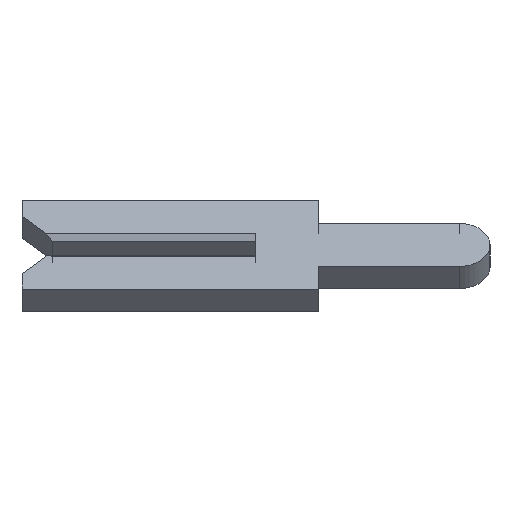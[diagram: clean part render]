
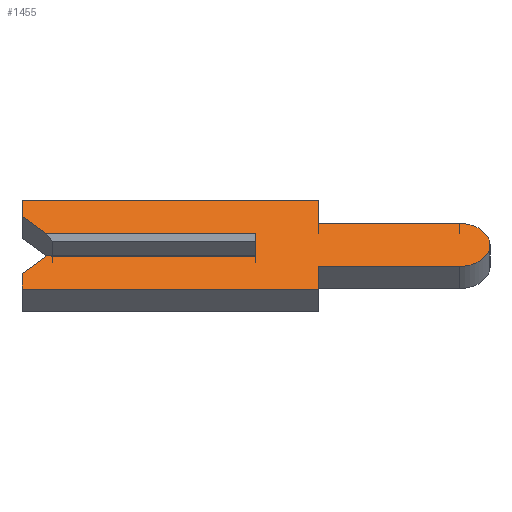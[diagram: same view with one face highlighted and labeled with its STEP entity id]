
A CAD part, left-side view. The second image highlights one B-rep face of the part: STEP entity #1455.
In plain terms, the highlighted face is planar.
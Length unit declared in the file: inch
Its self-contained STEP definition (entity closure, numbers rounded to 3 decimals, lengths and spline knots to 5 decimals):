
#9 = CARTESIAN_POINT ( 'NONE',  ( -0.01, 0.1305, 0.0065 ) ) ;
#16 = VERTEX_POINT ( 'NONE', #1752 ) ;
#35 = VECTOR ( 'NONE', #376, 39.37008 ) ;
#37 = CARTESIAN_POINT ( 'NONE',  ( -0.01, 0.134, 0.01 ) ) ;
#63 = DIRECTION ( 'NONE',  ( 0., -1., 0. ) ) ;
#74 = ORIENTED_EDGE ( 'NONE', *, *, #1383, .F. ) ;
#86 = CARTESIAN_POINT ( 'NONE',  ( -0.01, -0.04, -0.04 ) ) ;
#107 = EDGE_CURVE ( 'NONE', #1207, #773, #765, .T. ) ;
#119 = DIRECTION ( 'NONE',  ( 0., 0., 1. ) ) ;
#122 = AXIS2_PLACEMENT_3D ( 'NONE', #515, #1673, #805 ) ;
#140 = DIRECTION ( 'NONE',  ( 0., 0.707, 0.707 ) ) ;
#144 = CARTESIAN_POINT ( 'NONE',  ( -0.01, -0.04, 0.0195 ) ) ;
#207 = CARTESIAN_POINT ( 'NONE',  ( -0.01, 0.15, 0.026 ) ) ;
#211 = EDGE_CURVE ( 'NONE', #896, #400, #517, .T. ) ;
#214 = CARTESIAN_POINT ( 'NONE',  ( -0.01, 0.15, 0.01 ) ) ;
#222 = CARTESIAN_POINT ( 'NONE',  ( -0.01, -0.04, 0.0195 ) ) ;
#225 = LINE ( 'NONE', #992, #1012 ) ;
#232 = DIRECTION ( 'NONE',  ( 0., 0., -1. ) ) ;
#243 = VECTOR ( 'NONE', #232, 39.37008 ) ;
#244 = DIRECTION ( 'NONE',  ( 0., -0.707, 0.707 ) ) ;
#254 = ORIENTED_EDGE ( 'NONE', *, *, #1159, .F. ) ;
#257 = CARTESIAN_POINT ( 'NONE',  ( -0.01, 0.15, 0.04 ) ) ;
#262 = DIRECTION ( 'NONE',  ( 1., 0., 0. ) ) ;
#268 = VECTOR ( 'NONE', #952, 39.37008 ) ;
#288 = LINE ( 'NONE', #681, #630 ) ;
#320 = CARTESIAN_POINT ( 'NONE',  ( -0.01, 0.15, -0.026 ) ) ;
#349 = VERTEX_POINT ( 'NONE', #1772 ) ;
#360 = LINE ( 'NONE', #541, #1742 ) ;
#376 = DIRECTION ( 'NONE',  ( 0., 0., -1. ) ) ;
#378 = LINE ( 'NONE', #811, #268 ) ;
#397 = VECTOR ( 'NONE', #1154, 39.37008 ) ;
#400 = VERTEX_POINT ( 'NONE', #1021 ) ;
#404 = CARTESIAN_POINT ( 'NONE',  ( -0.01, -0.1305, 0. ) ) ;
#422 = LINE ( 'NONE', #795, #1818 ) ;
#462 = VERTEX_POINT ( 'NONE', #320 ) ;
#465 = VERTEX_POINT ( 'NONE', #1200 ) ;
#481 = CARTESIAN_POINT ( 'NONE',  ( -0.01, -0.04, -0.0195 ) ) ;
#515 = CARTESIAN_POINT ( 'NONE',  ( -0.01, -0.1305, 0. ) ) ;
#517 = LINE ( 'NONE', #9, #1617 ) ;
#521 = ORIENTED_EDGE ( 'NONE', *, *, #107, .F. ) ;
#541 = CARTESIAN_POINT ( 'NONE',  ( -0.01, 0.15, -0.026 ) ) ;
#549 = ORIENTED_EDGE ( 'NONE', *, *, #987, .T. ) ;
#559 = CARTESIAN_POINT ( 'NONE',  ( -0.01, -0.04, 0.04 ) ) ;
#609 = LINE ( 'NONE', #86, #243 ) ;
#623 = ORIENTED_EDGE ( 'NONE', *, *, #1677, .F. ) ;
#630 = VECTOR ( 'NONE', #997, 39.37008 ) ;
#668 = DIRECTION ( 'NONE',  ( 0., -1., 0. ) ) ;
#674 = LINE ( 'NONE', #222, #993 ) ;
#681 = CARTESIAN_POINT ( 'NONE',  ( -0.01, -0.04, -0.0195 ) ) ;
#692 = EDGE_LOOP ( 'NONE', ( #549, #1679, #749, #254, #623, #521, #959, #1429, #1628, #1826, #837, #74, #1052, #978 ) ) ;
#718 = VECTOR ( 'NONE', #244, 39.37008 ) ;
#720 = VECTOR ( 'NONE', #1498, 39.37008 ) ;
#749 = ORIENTED_EDGE ( 'NONE', *, *, #1249, .F. ) ;
#765 = LINE ( 'NONE', #1160, #397 ) ;
#773 = VERTEX_POINT ( 'NONE', #1509 ) ;
#792 = EDGE_CURVE ( 'NONE', #400, #1481, #830, .T. ) ;
#795 = CARTESIAN_POINT ( 'NONE',  ( -0.01, -0.1305, -0.01 ) ) ;
#805 = DIRECTION ( 'NONE',  ( 0., 0., -1. ) ) ;
#811 = CARTESIAN_POINT ( 'NONE',  ( -0.01, 0.15, 0.04 ) ) ;
#830 = LINE ( 'NONE', #207, #720 ) ;
#837 = ORIENTED_EDGE ( 'NONE', *, *, #1413, .F. ) ;
#863 = VERTEX_POINT ( 'NONE', #1655 ) ;
#896 = VERTEX_POINT ( 'NONE', #37 ) ;
#900 = LINE ( 'NONE', #1252, #35 ) ;
#912 = AXIS2_PLACEMENT_3D ( 'NONE', #404, #262, #1568 ) ;
#952 = DIRECTION ( 'NONE',  ( 0., -1., 0. ) ) ;
#956 = DIRECTION ( 'NONE',  ( 0., -1., 0. ) ) ;
#959 = ORIENTED_EDGE ( 'NONE', *, *, #1449, .F. ) ;
#978 = ORIENTED_EDGE ( 'NONE', *, *, #211, .F. ) ;
#987 = EDGE_CURVE ( 'NONE', #896, #1494, #1202, .T. ) ;
#992 = CARTESIAN_POINT ( 'NONE',  ( -0.01, 0., 0.0065 ) ) ;
#993 = VECTOR ( 'NONE', #668, 39.37008 ) ;
#997 = DIRECTION ( 'NONE',  ( 0., 1., 0. ) ) ;
#1012 = VECTOR ( 'NONE', #119, 39.37008 ) ;
#1021 = CARTESIAN_POINT ( 'NONE',  ( -0.01, 0.15, 0.026 ) ) ;
#1052 = ORIENTED_EDGE ( 'NONE', *, *, #792, .F. ) ;
#1079 = VECTOR ( 'NONE', #63, 39.37008 ) ;
#1097 = VERTEX_POINT ( 'NONE', #481 ) ;
#1153 = CIRCLE ( 'NONE', #122, 0.0195 ) ;
#1154 = DIRECTION ( 'NONE',  ( 0., 1., 0. ) ) ;
#1159 = EDGE_CURVE ( 'NONE', #462, #465, #1682, .T. ) ;
#1160 = CARTESIAN_POINT ( 'NONE',  ( -0.01, 0.15, -0.04 ) ) ;
#1170 = VERTEX_POINT ( 'NONE', #144 ) ;
#1200 = CARTESIAN_POINT ( 'NONE',  ( -0.01, 0.134, -0.01 ) ) ;
#1202 = LINE ( 'NONE', #214, #1079 ) ;
#1207 = VERTEX_POINT ( 'NONE', #1685 ) ;
#1222 = EDGE_CURVE ( 'NONE', #863, #349, #1153, .T. ) ;
#1249 = EDGE_CURVE ( 'NONE', #465, #16, #422, .T. ) ;
#1252 = CARTESIAN_POINT ( 'NONE',  ( -0.01, -0.04, 0.04 ) ) ;
#1383 = EDGE_CURVE ( 'NONE', #1481, #1686, #378, .T. ) ;
#1411 = PLANE ( 'NONE',  #912 ) ;
#1413 = EDGE_CURVE ( 'NONE', #1686, #1170, #900, .T. ) ;
#1429 = ORIENTED_EDGE ( 'NONE', *, *, #1583, .F. ) ;
#1434 = EDGE_CURVE ( 'NONE', #1170, #863, #674, .T. ) ;
#1449 = EDGE_CURVE ( 'NONE', #1097, #1207, #609, .T. ) ;
#1455 = ADVANCED_FACE ( 'NONE', ( #1797 ), #1411, .F. ) ;
#1481 = VERTEX_POINT ( 'NONE', #257 ) ;
#1494 = VERTEX_POINT ( 'NONE', #1726 ) ;
#1498 = DIRECTION ( 'NONE',  ( 0., 0., 1. ) ) ;
#1509 = CARTESIAN_POINT ( 'NONE',  ( -0.01, 0.15, -0.04 ) ) ;
#1519 = CARTESIAN_POINT ( 'NONE',  ( -0.01, 0.1305, -0.0065 ) ) ;
#1554 = EDGE_CURVE ( 'NONE', #16, #1494, #225, .T. ) ;
#1568 = DIRECTION ( 'NONE',  ( 0., 0., -1. ) ) ;
#1580 = DIRECTION ( 'NONE',  ( 0., 0., 1. ) ) ;
#1583 = EDGE_CURVE ( 'NONE', #349, #1097, #288, .T. ) ;
#1617 = VECTOR ( 'NONE', #140, 39.37008 ) ;
#1628 = ORIENTED_EDGE ( 'NONE', *, *, #1222, .F. ) ;
#1655 = CARTESIAN_POINT ( 'NONE',  ( -0.01, -0.1305, 0.0195 ) ) ;
#1673 = DIRECTION ( 'NONE',  ( 1., 0., 0. ) ) ;
#1677 = EDGE_CURVE ( 'NONE', #773, #462, #360, .T. ) ;
#1679 = ORIENTED_EDGE ( 'NONE', *, *, #1554, .F. ) ;
#1682 = LINE ( 'NONE', #1519, #718 ) ;
#1685 = CARTESIAN_POINT ( 'NONE',  ( -0.01, -0.04, -0.04 ) ) ;
#1686 = VERTEX_POINT ( 'NONE', #559 ) ;
#1726 = CARTESIAN_POINT ( 'NONE',  ( -0.01, 0., 0.01 ) ) ;
#1742 = VECTOR ( 'NONE', #1580, 39.37008 ) ;
#1752 = CARTESIAN_POINT ( 'NONE',  ( -0.01, 0., -0.01 ) ) ;
#1772 = CARTESIAN_POINT ( 'NONE',  ( -0.01, -0.1305, -0.0195 ) ) ;
#1797 = FACE_OUTER_BOUND ( 'NONE', #692, .T. ) ;
#1818 = VECTOR ( 'NONE', #956, 39.37008 ) ;
#1826 = ORIENTED_EDGE ( 'NONE', *, *, #1434, .F. ) ;
